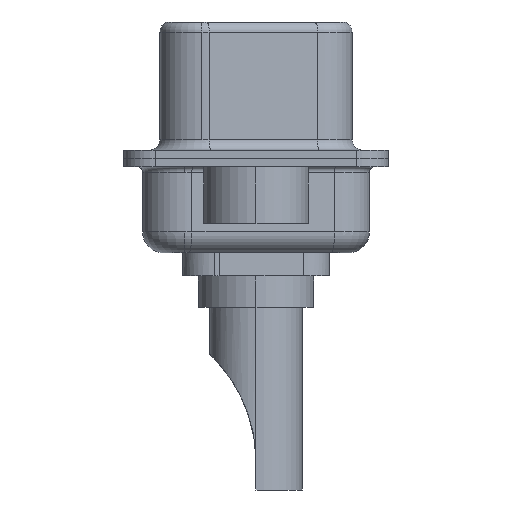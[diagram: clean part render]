
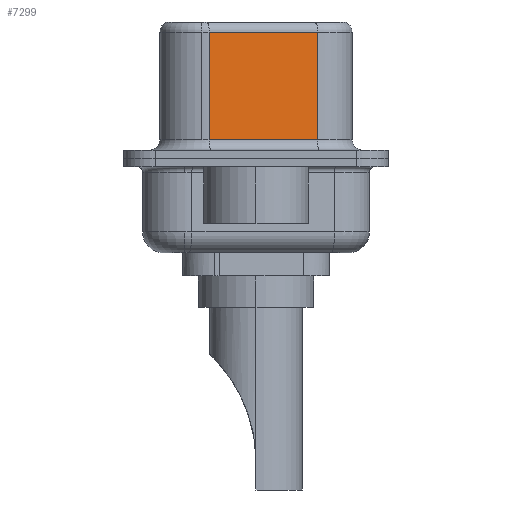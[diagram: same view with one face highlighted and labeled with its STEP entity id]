
A CAD part, left-side view. The second image highlights one B-rep face of the part: STEP entity #7299.
In plain terms, the highlighted planar face has unit normal (-0.985, -0.174, 0).
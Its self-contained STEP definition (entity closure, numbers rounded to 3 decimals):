
#485 = VECTOR ( 'NONE', #11540, 1000. ) ;
#1354 = VECTOR ( 'NONE', #12589, 1000. ) ;
#1930 = EDGE_CURVE ( 'NONE', #2132, #13509, #12568, .T. ) ;
#2128 = DIRECTION ( 'NONE',  ( -0.174, 0.985, 0. ) ) ;
#2132 = VERTEX_POINT ( 'NONE', #4215 ) ;
#3258 = CARTESIAN_POINT ( 'NONE',  ( 3.675, 2.233, 0.9 ) ) ;
#3350 = DIRECTION ( 'NONE',  ( 0.985, 0.174, 0. ) ) ;
#3472 = ORIENTED_EDGE ( 'NONE', *, *, #1930, .T. ) ;
#3616 = ORIENTED_EDGE ( 'NONE', *, *, #8334, .T. ) ;
#3995 = LINE ( 'NONE', #7181, #485 ) ;
#4098 = LINE ( 'NONE', #7018, #12897 ) ;
#4215 = CARTESIAN_POINT ( 'NONE',  ( 4.585, -2.927, 6.02 ) ) ;
#4476 = VECTOR ( 'NONE', #4496, 1000. ) ;
#4496 = DIRECTION ( 'NONE',  ( -0.174, 0.985, 0. ) ) ;
#4498 = LINE ( 'NONE', #9365, #1354 ) ;
#4942 = CARTESIAN_POINT ( 'NONE',  ( 4.585, -2.927, 6.52 ) ) ;
#5024 = CARTESIAN_POINT ( 'NONE',  ( 4.585, -2.927, 0.9 ) ) ;
#6223 = CARTESIAN_POINT ( 'NONE',  ( 3.675, 2.233, 6.02 ) ) ;
#6631 = EDGE_LOOP ( 'NONE', ( #12941, #3472, #3616, #13286 ) ) ;
#7018 = CARTESIAN_POINT ( 'NONE',  ( 4.585, -2.927, 6.52 ) ) ;
#7181 = CARTESIAN_POINT ( 'NONE',  ( 4.585, -2.927, 0.9 ) ) ;
#7299 = ADVANCED_FACE ( 'NONE', ( #10473 ), #14059, .F. ) ;
#7674 = EDGE_CURVE ( 'NONE', #10616, #12515, #3995, .T. ) ;
#8131 = DIRECTION ( 'NONE',  ( 0., 0., -1. ) ) ;
#8334 = EDGE_CURVE ( 'NONE', #13509, #10616, #4498, .T. ) ;
#9365 = CARTESIAN_POINT ( 'NONE',  ( 3.675, 2.233, 6.52 ) ) ;
#10073 = AXIS2_PLACEMENT_3D ( 'NONE', #4942, #3350, #2128 ) ;
#10473 = FACE_OUTER_BOUND ( 'NONE', #6631, .T. ) ;
#10616 = VERTEX_POINT ( 'NONE', #3258 ) ;
#11540 = DIRECTION ( 'NONE',  ( 0.174, -0.985, 0. ) ) ;
#11706 = EDGE_CURVE ( 'NONE', #2132, #12515, #4098, .T. ) ;
#11830 = CARTESIAN_POINT ( 'NONE',  ( 4.585, -2.927, 6.02 ) ) ;
#12515 = VERTEX_POINT ( 'NONE', #5024 ) ;
#12568 = LINE ( 'NONE', #11830, #4476 ) ;
#12589 = DIRECTION ( 'NONE',  ( 0., 0., -1. ) ) ;
#12897 = VECTOR ( 'NONE', #8131, 1000. ) ;
#12941 = ORIENTED_EDGE ( 'NONE', *, *, #11706, .F. ) ;
#13286 = ORIENTED_EDGE ( 'NONE', *, *, #7674, .T. ) ;
#13509 = VERTEX_POINT ( 'NONE', #6223 ) ;
#14059 = PLANE ( 'NONE',  #10073 ) ;
